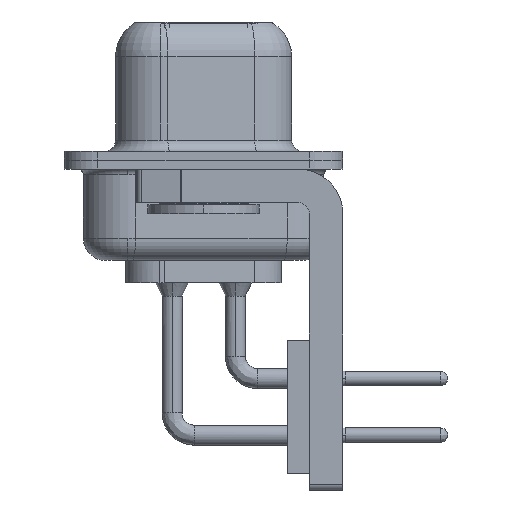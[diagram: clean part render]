
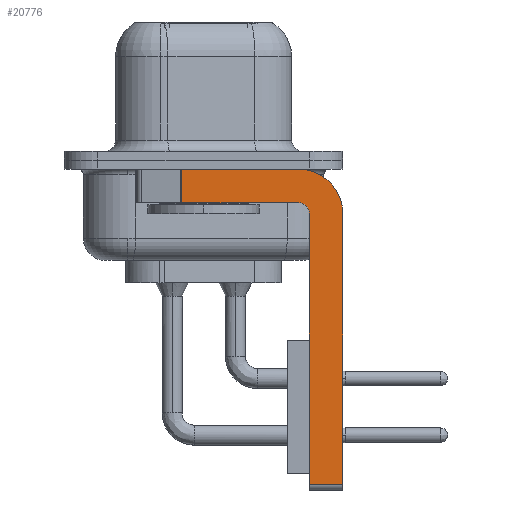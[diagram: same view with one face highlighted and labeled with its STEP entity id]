
A CAD part, left-side view. The second image highlights one B-rep face of the part: STEP entity #20776.
In plain terms, the highlighted planar face has unit normal (-1, 0, 0).
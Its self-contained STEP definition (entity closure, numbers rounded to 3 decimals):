
#586 = ORIENTED_EDGE ( 'NONE', *, *, #19774, .F. ) ;
#1935 = AXIS2_PLACEMENT_3D ( 'NONE', #10455, #17489, #3429 ) ;
#1979 = LINE ( 'NONE', #25134, #13066 ) ;
#2486 = CARTESIAN_POINT ( 'NONE',  ( -2.9, -4.25, -1.9 ) ) ;
#2997 = ORIENTED_EDGE ( 'NONE', *, *, #13083, .T. ) ;
#3429 = DIRECTION ( 'NONE',  ( 0., 0., -1. ) ) ;
#4291 = CARTESIAN_POINT ( 'NONE',  ( -2.9, -6.25, -2.4 ) ) ;
#4470 = DIRECTION ( 'NONE',  ( 0., -1., 0. ) ) ;
#4728 = DIRECTION ( 'NONE',  ( -1., 0., 0. ) ) ;
#4857 = ORIENTED_EDGE ( 'NONE', *, *, #26467, .F. ) ;
#5796 = LINE ( 'NONE', #2486, #17497 ) ;
#6083 = CARTESIAN_POINT ( 'NONE',  ( -2.9, -4.75, -14.55 ) ) ;
#6096 = CARTESIAN_POINT ( 'NONE',  ( -2.9, -4.25, -2.4 ) ) ;
#6817 = ORIENTED_EDGE ( 'NONE', *, *, #18778, .F. ) ;
#7261 = AXIS2_PLACEMENT_3D ( 'NONE', #6096, #22392, #8412 ) ;
#7945 = VERTEX_POINT ( 'NONE', #30346 ) ;
#7972 = ORIENTED_EDGE ( 'NONE', *, *, #24067, .F. ) ;
#8383 = VECTOR ( 'NONE', #8772, 1000. ) ;
#8412 = DIRECTION ( 'NONE',  ( 0., 0., -1. ) ) ;
#8533 = VERTEX_POINT ( 'NONE', #18281 ) ;
#8772 = DIRECTION ( 'NONE',  ( 0., 0., 1. ) ) ;
#8910 = VECTOR ( 'NONE', #16097, 1000. ) ;
#8951 = DIRECTION ( 'NONE',  ( 0., 0., -1. ) ) ;
#9099 = CARTESIAN_POINT ( 'NONE',  ( -2.9, -4.25, -14.55 ) ) ;
#9490 = CARTESIAN_POINT ( 'NONE',  ( -2.9, -4.75, -2.4 ) ) ;
#10162 = ORIENTED_EDGE ( 'NONE', *, *, #29444, .F. ) ;
#10455 = CARTESIAN_POINT ( 'NONE',  ( -2.9, -4.25, -2.4 ) ) ;
#13066 = VECTOR ( 'NONE', #22701, 1000. ) ;
#13068 = CIRCLE ( 'NONE', #7261, 2. ) ;
#13083 = EDGE_CURVE ( 'NONE', #7945, #28047, #15466, .T. ) ;
#13155 = CIRCLE ( 'NONE', #17796, 0.5 ) ;
#13755 = CARTESIAN_POINT ( 'NONE',  ( -2.9, 3., -0.4 ) ) ;
#14262 = DIRECTION ( 'NONE',  ( 0., 1., 0. ) ) ;
#14293 = EDGE_CURVE ( 'NONE', #29224, #26547, #29791, .T. ) ;
#14328 = CARTESIAN_POINT ( 'NONE',  ( -2.9, -4.25, -1.9 ) ) ;
#14401 = VERTEX_POINT ( 'NONE', #14328 ) ;
#14638 = LINE ( 'NONE', #15745, #8383 ) ;
#15267 = ORIENTED_EDGE ( 'NONE', *, *, #24818, .F. ) ;
#15466 = LINE ( 'NONE', #20564, #21616 ) ;
#15745 = CARTESIAN_POINT ( 'NONE',  ( -2.9, -4.75, -14.8 ) ) ;
#16097 = DIRECTION ( 'NONE',  ( 0., -1., 0. ) ) ;
#17489 = DIRECTION ( 'NONE',  ( 1., 0., 0. ) ) ;
#17497 = VECTOR ( 'NONE', #14262, 1000. ) ;
#17796 = AXIS2_PLACEMENT_3D ( 'NONE', #18740, #4728, #21069 ) ;
#18281 = CARTESIAN_POINT ( 'NONE',  ( -2.9, -4.25, -0.4 ) ) ;
#18740 = CARTESIAN_POINT ( 'NONE',  ( -2.9, -4.25, -2.4 ) ) ;
#18778 = EDGE_CURVE ( 'NONE', #14401, #28047, #5796, .T. ) ;
#19774 = EDGE_CURVE ( 'NONE', #27532, #26547, #1979, .T. ) ;
#20564 = CARTESIAN_POINT ( 'NONE',  ( -2.9, 0.978, -1.9 ) ) ;
#20776 = ADVANCED_FACE ( 'NONE', ( #26979 ), #29140, .F. ) ;
#21069 = DIRECTION ( 'NONE',  ( 0., 0., 1. ) ) ;
#21293 = LINE ( 'NONE', #13755, #8910 ) ;
#21314 = ORIENTED_EDGE ( 'NONE', *, *, #14293, .T. ) ;
#21616 = VECTOR ( 'NONE', #8951, 1000. ) ;
#21689 = EDGE_LOOP ( 'NONE', ( #10162, #2997, #6817, #15267, #7972, #21314, #586, #4857 ) ) ;
#22392 = DIRECTION ( 'NONE',  ( 1., 0., 0. ) ) ;
#22701 = DIRECTION ( 'NONE',  ( 0., 0., -1. ) ) ;
#23419 = VECTOR ( 'NONE', #4470, 1000. ) ;
#24067 = EDGE_CURVE ( 'NONE', #29224, #28310, #14638, .T. ) ;
#24818 = EDGE_CURVE ( 'NONE', #28310, #14401, #13155, .T. ) ;
#25134 = CARTESIAN_POINT ( 'NONE',  ( -2.9, -6.25, -2.4 ) ) ;
#26467 = EDGE_CURVE ( 'NONE', #8533, #27532, #13068, .T. ) ;
#26547 = VERTEX_POINT ( 'NONE', #28905 ) ;
#26979 = FACE_OUTER_BOUND ( 'NONE', #21689, .T. ) ;
#27532 = VERTEX_POINT ( 'NONE', #4291 ) ;
#28047 = VERTEX_POINT ( 'NONE', #29678 ) ;
#28310 = VERTEX_POINT ( 'NONE', #9490 ) ;
#28905 = CARTESIAN_POINT ( 'NONE',  ( -2.9, -6.25, -14.55 ) ) ;
#29140 = PLANE ( 'NONE',  #1935 ) ;
#29224 = VERTEX_POINT ( 'NONE', #6083 ) ;
#29444 = EDGE_CURVE ( 'NONE', #7945, #8533, #21293, .T. ) ;
#29678 = CARTESIAN_POINT ( 'NONE',  ( -2.9, 0.978, -1.9 ) ) ;
#29791 = LINE ( 'NONE', #9099, #23419 ) ;
#30346 = CARTESIAN_POINT ( 'NONE',  ( -2.9, 0.978, -0.4 ) ) ;
